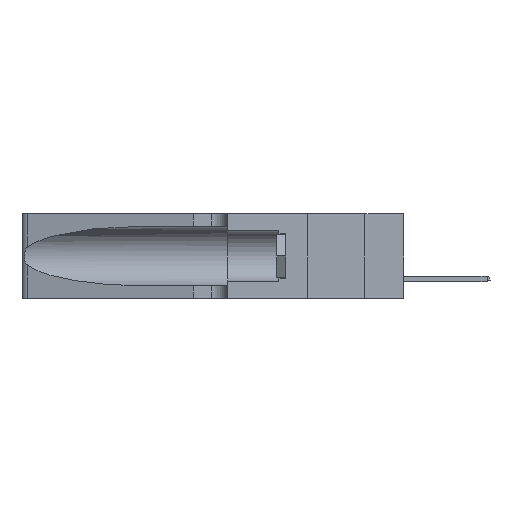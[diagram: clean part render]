
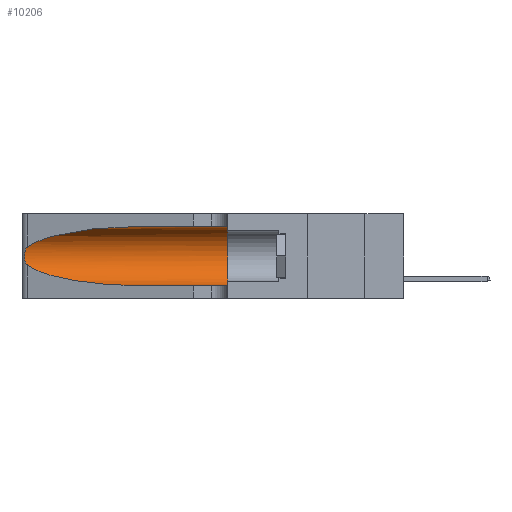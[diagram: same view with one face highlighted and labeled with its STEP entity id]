
A CAD part, left-side view. The second image highlights one B-rep face of the part: STEP entity #10206.
In plain terms, the highlighted cylindrical face has radius 3.308 mm (diameter 6.617 mm), a partial arc.
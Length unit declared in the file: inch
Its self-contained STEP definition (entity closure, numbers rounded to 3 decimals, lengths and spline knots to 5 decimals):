
#599 = CARTESIAN_POINT ( 'NONE',  ( 0.1305, 1.61858, 0.05475 ) ) ;
#2188 = AXIS2_PLACEMENT_3D ( 'NONE', #25165, #46983, #10717 ) ;
#2486 = EDGE_CURVE ( 'NONE', #16634, #45805, #12247, .T. ) ;
#2643 = CARTESIAN_POINT ( 'NONE',  ( 0.1305, 0.35, 0.05475 ) ) ;
#7204 = CARTESIAN_POINT ( 'NONE',  ( 0.25487, 1.22718, 0.14631 ) ) ;
#7265 = DIRECTION ( 'NONE',  ( 0., -1., 0. ) ) ;
#7479 = VERTEX_POINT ( 'NONE', #33685 ) ;
#7494 = DIRECTION ( 'NONE',  ( 0., -1., 0. ) ) ;
#7668 = CARTESIAN_POINT ( 'NONE',  ( 0.25789, 1.23486, 0.15765 ) ) ;
#7832 = CARTESIAN_POINT ( 'NONE',  ( 0.25639, 1.23184, 0.21858 ) ) ;
#8572 = EDGE_CURVE ( 'NONE', #46036, #45805, #29454, .T. ) ;
#10206 = ADVANCED_FACE ( 'NONE', ( #28745 ), #18996, .F. ) ;
#10605 = EDGE_CURVE ( 'NONE', #23460, #46036, #17334, .T. ) ;
#10689 = ORIENTED_EDGE ( 'NONE', *, *, #18572, .F. ) ;
#10717 = DIRECTION ( 'NONE',  ( 0., 0., 1. ) ) ;
#10854 = CARTESIAN_POINT ( 'NONE',  ( 0.25856, 1.23593, 0.16098 ) ) ;
#11014 = CARTESIAN_POINT ( 'NONE',  ( 0.25555, 1.22994, 0.2215 ) ) ;
#11609 = CARTESIAN_POINT ( 'NONE',  ( 0.1305, 0.35, 0.31525 ) ) ;
#11977 = VERTEX_POINT ( 'NONE', #35884 ) ;
#12247 = CIRCLE ( 'NONE', #2188, 0.13025 ) ;
#12336 =( BOUNDED_CURVE ( )  B_SPLINE_CURVE ( 3, ( #33540, #44788, #15259, #33706 ),
 .UNSPECIFIED., .F., .F. ) 
 B_SPLINE_CURVE_WITH_KNOTS ( ( 4, 4 ),
 ( 1.5708, 2.84003 ),
 .UNSPECIFIED. ) 
 CURVE ( )  GEOMETRIC_REPRESENTATION_ITEM ( )  RATIONAL_B_SPLINE_CURVE ( ( 1., 0.87, 0.87, 1. ) ) 
 REPRESENTATION_ITEM ( '' )  );
#13933 = VECTOR ( 'NONE', #7494, 39.37008 ) ;
#13950 = ORIENTED_EDGE ( 'NONE', *, *, #10605, .T. ) ;
#14713 = CARTESIAN_POINT ( 'NONE',  ( 0.1305, 0.72297, 0.05475 ) ) ;
#15259 = CARTESIAN_POINT ( 'NONE',  ( 0.2373, 1.15595, 0.28018 ) ) ;
#16634 = VERTEX_POINT ( 'NONE', #11609 ) ;
#17334 =( BOUNDED_CURVE ( )  B_SPLINE_CURVE ( 3, ( #7204, #21793, #25475, #14713 ),
 .UNSPECIFIED., .F., .T. ) 
 B_SPLINE_CURVE_WITH_KNOTS ( ( 4, 4 ),
 ( 3.44316, 4.71239 ),
 .UNSPECIFIED. ) 
 CURVE ( )  GEOMETRIC_REPRESENTATION_ITEM ( )  RATIONAL_B_SPLINE_CURVE ( ( 1., 0.87, 0.87, 1. ) ) 
 REPRESENTATION_ITEM ( '' )  );
#18252 = CARTESIAN_POINT ( 'NONE',  ( 0.25487, 1.22718, 0.22369 ) ) ;
#18320 = CARTESIAN_POINT ( 'NONE',  ( 0.1305, 1.61858, 0.185 ) ) ;
#18572 = EDGE_CURVE ( 'NONE', #7479, #16634, #47034, .T. ) ;
#18858 = EDGE_LOOP ( 'NONE', ( #26779, #27459, #13950, #19982, #36577, #10689 ) ) ;
#18996 = CYLINDRICAL_SURFACE ( 'NONE', #34555, 0.13025 ) ;
#19223 = DIRECTION ( 'NONE',  ( 0., -1., 0. ) ) ;
#19982 = ORIENTED_EDGE ( 'NONE', *, *, #8572, .T. ) ;
#21793 = CARTESIAN_POINT ( 'NONE',  ( 0.2373, 1.15595, 0.08982 ) ) ;
#22256 = CARTESIAN_POINT ( 'NONE',  ( 0.25787, 1.23484, 0.2124 ) ) ;
#22921 = VECTOR ( 'NONE', #19223, 39.37008 ) ;
#23460 = VERTEX_POINT ( 'NONE', #29406 ) ;
#25165 = CARTESIAN_POINT ( 'NONE',  ( 0.1305, 0.35, 0.185 ) ) ;
#25475 = CARTESIAN_POINT ( 'NONE',  ( 0.18966, 0.96281, 0.05475 ) ) ;
#25881 = B_SPLINE_CURVE_WITH_KNOTS ( 'NONE', 3,
 ( #18252, #11014, #7832, #22256, #26119, #29780, #33164, #44558, #33000, #10854, #7668, #40659, #33472, #40182 ),
 .UNSPECIFIED., .F., .F.,
 ( 4, 2, 2, 2, 2, 2, 4 ),
 ( 0., 0.00027, 0.00053, 0.00107, 0.0016, 0.00187, 0.00214 ),
 .UNSPECIFIED. ) ;
#26119 = CARTESIAN_POINT ( 'NONE',  ( 0.25854, 1.2359, 0.20912 ) ) ;
#26779 = ORIENTED_EDGE ( 'NONE', *, *, #35423, .T. ) ;
#26925 = CARTESIAN_POINT ( 'NONE',  ( 0.1305, 1.61858, 0.31525 ) ) ;
#27459 = ORIENTED_EDGE ( 'NONE', *, *, #43346, .T. ) ;
#28745 = FACE_OUTER_BOUND ( 'NONE', #18858, .T. ) ;
#29406 = CARTESIAN_POINT ( 'NONE',  ( 0.25487, 1.22718, 0.14631 ) ) ;
#29454 = LINE ( 'NONE', #599, #13933 ) ;
#29527 = DIRECTION ( 'NONE',  ( 0., 0., -1. ) ) ;
#29780 = CARTESIAN_POINT ( 'NONE',  ( 0.26018, 1.23835, 0.19895 ) ) ;
#33000 = CARTESIAN_POINT ( 'NONE',  ( 0.26017, 1.23833, 0.17102 ) ) ;
#33164 = CARTESIAN_POINT ( 'NONE',  ( 0.26075, 1.23896, 0.19203 ) ) ;
#33472 = CARTESIAN_POINT ( 'NONE',  ( 0.25555, 1.22993, 0.14849 ) ) ;
#33540 = CARTESIAN_POINT ( 'NONE',  ( 0.1305, 0.72297, 0.31525 ) ) ;
#33685 = CARTESIAN_POINT ( 'NONE',  ( 0.1305, 0.72297, 0.31525 ) ) ;
#33706 = CARTESIAN_POINT ( 'NONE',  ( 0.25487, 1.22718, 0.22369 ) ) ;
#34555 = AXIS2_PLACEMENT_3D ( 'NONE', #18320, #7265, #29527 ) ;
#35423 = EDGE_CURVE ( 'NONE', #7479, #11977, #12336, .T. ) ;
#35884 = CARTESIAN_POINT ( 'NONE',  ( 0.25487, 1.22718, 0.22369 ) ) ;
#36577 = ORIENTED_EDGE ( 'NONE', *, *, #2486, .F. ) ;
#40182 = CARTESIAN_POINT ( 'NONE',  ( 0.25487, 1.22718, 0.14631 ) ) ;
#40659 = CARTESIAN_POINT ( 'NONE',  ( 0.25639, 1.23186, 0.15144 ) ) ;
#43346 = EDGE_CURVE ( 'NONE', #11977, #23460, #25881, .T. ) ;
#44558 = CARTESIAN_POINT ( 'NONE',  ( 0.26075, 1.23896, 0.178 ) ) ;
#44788 = CARTESIAN_POINT ( 'NONE',  ( 0.18966, 0.96281, 0.31525 ) ) ;
#45805 = VERTEX_POINT ( 'NONE', #2643 ) ;
#46036 = VERTEX_POINT ( 'NONE', #47014 ) ;
#46983 = DIRECTION ( 'NONE',  ( 0., 1., 0. ) ) ;
#47014 = CARTESIAN_POINT ( 'NONE',  ( 0.1305, 0.72297, 0.05475 ) ) ;
#47034 = LINE ( 'NONE', #26925, #22921 ) ;
